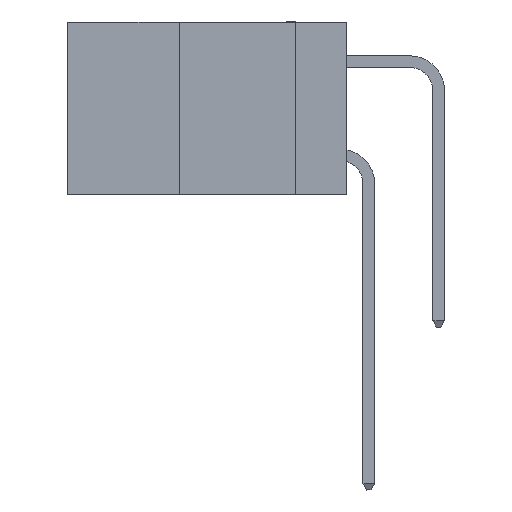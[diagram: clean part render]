
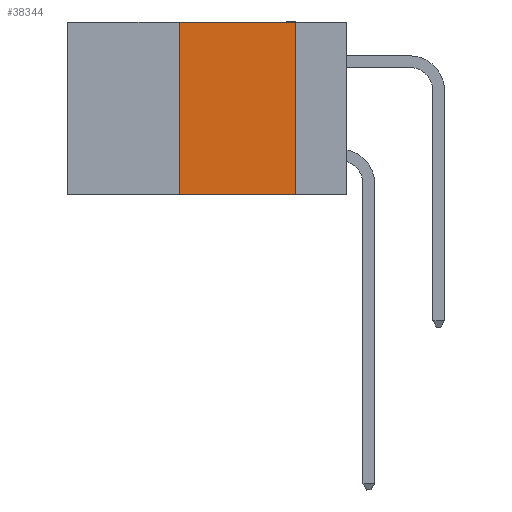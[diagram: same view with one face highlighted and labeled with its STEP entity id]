
A CAD part, left-side view. The second image highlights one B-rep face of the part: STEP entity #38344.
In plain terms, the highlighted planar face has unit normal (-1, 0, 0).
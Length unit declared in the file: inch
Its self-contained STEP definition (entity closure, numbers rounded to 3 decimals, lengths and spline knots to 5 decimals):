
#1944 = EDGE_CURVE ( 'NONE', #40003, #20044, #7600, .T. ) ;
#2551 = ORIENTED_EDGE ( 'NONE', *, *, #36081, .F. ) ;
#2746 = DIRECTION ( 'NONE',  ( 0., -1., 0. ) ) ;
#5004 = EDGE_CURVE ( 'NONE', #14984, #40003, #6787, .T. ) ;
#5907 = CARTESIAN_POINT ( 'NONE',  ( 0., 0.6, -0.37 ) ) ;
#6787 = LINE ( 'NONE', #32148, #30538 ) ;
#7600 = LINE ( 'NONE', #34907, #31359 ) ;
#8447 = DIRECTION ( 'NONE',  ( 0., 0., -1. ) ) ;
#9567 = DIRECTION ( 'NONE',  ( 0., -1., 0. ) ) ;
#10072 = CARTESIAN_POINT ( 'NONE',  ( 0., 0.11, 0. ) ) ;
#12845 = LINE ( 'NONE', #5907, #29044 ) ;
#13256 = ORIENTED_EDGE ( 'NONE', *, *, #27512, .T. ) ;
#14984 = VERTEX_POINT ( 'NONE', #17630 ) ;
#15863 = CARTESIAN_POINT ( 'NONE',  ( 0., 0.36, 0. ) ) ;
#17630 = CARTESIAN_POINT ( 'NONE',  ( 0., 0.36, 0. ) ) ;
#18062 = CARTESIAN_POINT ( 'NONE',  ( 0., 0.6, 0. ) ) ;
#18888 = DIRECTION ( 'NONE',  ( 0., 0., -1. ) ) ;
#19119 = DIRECTION ( 'NONE',  ( 0., 0., 1. ) ) ;
#20044 = VERTEX_POINT ( 'NONE', #22222 ) ;
#22222 = CARTESIAN_POINT ( 'NONE',  ( 0., 0.11, -0.37 ) ) ;
#24726 = VERTEX_POINT ( 'NONE', #36990 ) ;
#26411 = FACE_OUTER_BOUND ( 'NONE', #28452, .T. ) ;
#27424 = ORIENTED_EDGE ( 'NONE', *, *, #5004, .F. ) ;
#27512 = EDGE_CURVE ( 'NONE', #24726, #20044, #12845, .T. ) ;
#27804 = DIRECTION ( 'NONE',  ( 1., 0., 0. ) ) ;
#28452 = EDGE_LOOP ( 'NONE', ( #32952, #27424, #2551, #13256 ) ) ;
#29044 = VECTOR ( 'NONE', #2746, 39.37008 ) ;
#30052 = AXIS2_PLACEMENT_3D ( 'NONE', #18062, #27804, #8447 ) ;
#30538 = VECTOR ( 'NONE', #9567, 39.37008 ) ;
#31359 = VECTOR ( 'NONE', #18888, 39.37008 ) ;
#32148 = CARTESIAN_POINT ( 'NONE',  ( 0., 0.6, 0. ) ) ;
#32952 = ORIENTED_EDGE ( 'NONE', *, *, #1944, .F. ) ;
#34115 = PLANE ( 'NONE',  #30052 ) ;
#34907 = CARTESIAN_POINT ( 'NONE',  ( 0., 0.11, 0. ) ) ;
#36081 = EDGE_CURVE ( 'NONE', #24726, #14984, #37509, .T. ) ;
#36522 = VECTOR ( 'NONE', #19119, 39.37008 ) ;
#36990 = CARTESIAN_POINT ( 'NONE',  ( 0., 0.36, -0.37 ) ) ;
#37509 = LINE ( 'NONE', #15863, #36522 ) ;
#38344 = ADVANCED_FACE ( 'NONE', ( #26411 ), #34115, .F. ) ;
#40003 = VERTEX_POINT ( 'NONE', #10072 ) ;
